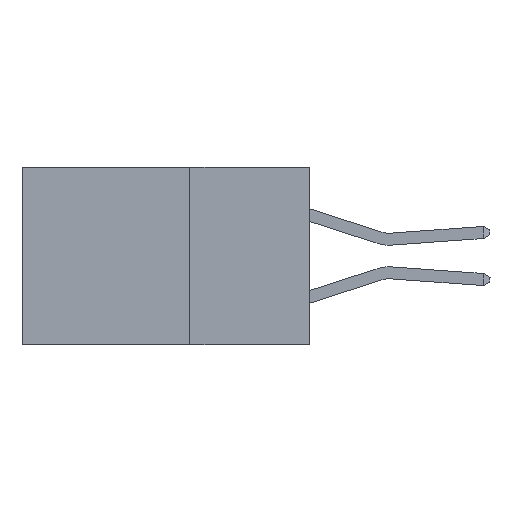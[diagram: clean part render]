
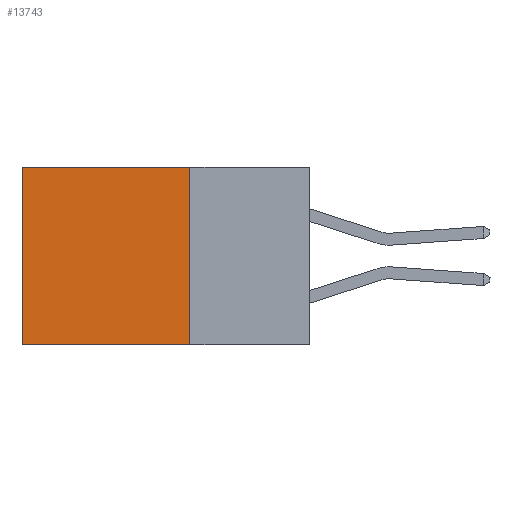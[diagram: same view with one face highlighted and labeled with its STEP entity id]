
A CAD part, left-side view. The second image highlights one B-rep face of the part: STEP entity #13743.
In plain terms, the highlighted planar face has unit normal (-1, 0, 0).
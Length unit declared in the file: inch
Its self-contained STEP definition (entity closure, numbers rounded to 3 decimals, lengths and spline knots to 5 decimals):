
#112 = VECTOR ( 'NONE', #12952, 39.37008 ) ;
#1479 = LINE ( 'NONE', #5359, #6540 ) ;
#1544 = VERTEX_POINT ( 'NONE', #18282 ) ;
#3174 = CARTESIAN_POINT ( 'NONE',  ( 0.298, 0.25, 0. ) ) ;
#3396 = PLANE ( 'NONE',  #3840 ) ;
#3656 = DIRECTION ( 'NONE',  ( 1., 0., 0. ) ) ;
#3840 = AXIS2_PLACEMENT_3D ( 'NONE', #18659, #3656, #14665 ) ;
#4160 = ORIENTED_EDGE ( 'NONE', *, *, #10880, .F. ) ;
#5359 = CARTESIAN_POINT ( 'NONE',  ( 0.298, 0.25, 0. ) ) ;
#5716 = VERTEX_POINT ( 'NONE', #11960 ) ;
#6115 = LINE ( 'NONE', #12887, #13253 ) ;
#6540 = VECTOR ( 'NONE', #18643, 39.37008 ) ;
#6753 = ORIENTED_EDGE ( 'NONE', *, *, #9358, .F. ) ;
#6822 = CARTESIAN_POINT ( 'NONE',  ( 0.298, 0.6, 0. ) ) ;
#8866 = CARTESIAN_POINT ( 'NONE',  ( 0.298, 0.6, 0. ) ) ;
#9358 = EDGE_CURVE ( 'NONE', #13581, #1544, #13301, .T. ) ;
#10880 = EDGE_CURVE ( 'NONE', #1544, #5716, #6115, .T. ) ;
#11252 = EDGE_CURVE ( 'NONE', #12121, #5716, #13925, .T. ) ;
#11671 = EDGE_CURVE ( 'NONE', #13581, #12121, #1479, .T. ) ;
#11960 = CARTESIAN_POINT ( 'NONE',  ( 0.298, 0.6, -0.37 ) ) ;
#12121 = VERTEX_POINT ( 'NONE', #8866 ) ;
#12887 = CARTESIAN_POINT ( 'NONE',  ( 0.298, 0.25, -0.37 ) ) ;
#12952 = DIRECTION ( 'NONE',  ( 0., 0., -1. ) ) ;
#13253 = VECTOR ( 'NONE', #15649, 39.37008 ) ;
#13301 = LINE ( 'NONE', #16258, #16521 ) ;
#13581 = VERTEX_POINT ( 'NONE', #3174 ) ;
#13743 = ADVANCED_FACE ( 'NONE', ( #16813 ), #3396, .F. ) ;
#13925 = LINE ( 'NONE', #6822, #112 ) ;
#14665 = DIRECTION ( 'NONE',  ( 0., 0., -1. ) ) ;
#14834 = ORIENTED_EDGE ( 'NONE', *, *, #11671, .T. ) ;
#15044 = ORIENTED_EDGE ( 'NONE', *, *, #11252, .T. ) ;
#15596 = EDGE_LOOP ( 'NONE', ( #15044, #4160, #6753, #14834 ) ) ;
#15649 = DIRECTION ( 'NONE',  ( 0., 1., 0. ) ) ;
#16258 = CARTESIAN_POINT ( 'NONE',  ( 0.298, 0.25, 0. ) ) ;
#16456 = DIRECTION ( 'NONE',  ( 0., 0., -1. ) ) ;
#16521 = VECTOR ( 'NONE', #16456, 39.37008 ) ;
#16813 = FACE_OUTER_BOUND ( 'NONE', #15596, .T. ) ;
#18282 = CARTESIAN_POINT ( 'NONE',  ( 0.298, 0.25, -0.37 ) ) ;
#18643 = DIRECTION ( 'NONE',  ( 0., 1., 0. ) ) ;
#18659 = CARTESIAN_POINT ( 'NONE',  ( 0.298, 0.25, 0. ) ) ;
